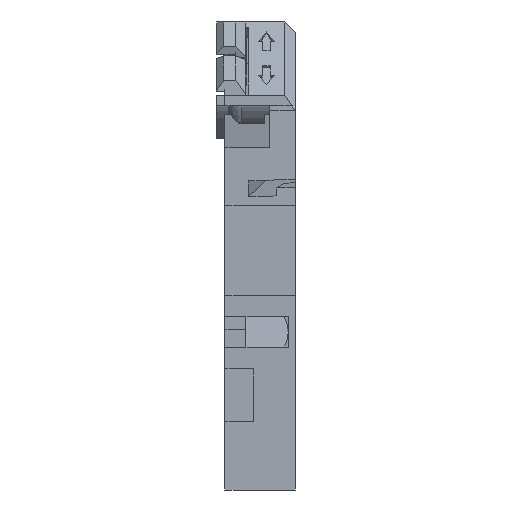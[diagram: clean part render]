
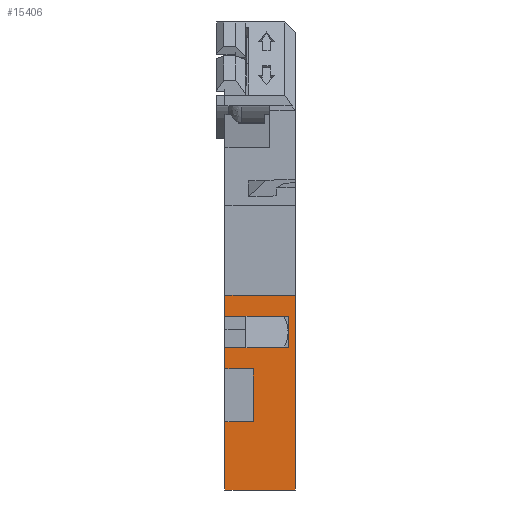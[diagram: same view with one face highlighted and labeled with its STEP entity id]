
A CAD part, left-side view. The second image highlights one B-rep face of the part: STEP entity #15406.
In plain terms, the highlighted planar face has unit normal (-1, 0, 0).
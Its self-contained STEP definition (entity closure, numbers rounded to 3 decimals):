
#14422 = VERTEX_POINT('',#14423);
#14423 = CARTESIAN_POINT('',(-50.,-1.6,-40.));
#14429 = EDGE_CURVE('',#14422,#14430,#14432,.T.);
#14430 = VERTEX_POINT('',#14431);
#14431 = CARTESIAN_POINT('',(-50.,-1.6,-27.));
#14432 = LINE('',#14433,#14434);
#14433 = CARTESIAN_POINT('',(-50.,-1.6,-40.));
#14434 = VECTOR('',#14435,1.);
#14435 = DIRECTION('',(0.,0.,1.));
#14454 = VERTEX_POINT('',#14455);
#14455 = CARTESIAN_POINT('',(-50.,-1.6,-17.));
#14461 = EDGE_CURVE('',#14462,#14454,#14464,.T.);
#14462 = VERTEX_POINT('',#14463);
#14463 = CARTESIAN_POINT('',(-50.,-1.6,-13.));
#14464 = LINE('',#14465,#14466);
#14465 = CARTESIAN_POINT('',(-50.,-1.6,-13.));
#14466 = VECTOR('',#14467,1.);
#14467 = DIRECTION('',(0.,0.,-1.));
#15386 = EDGE_CURVE('',#14422,#15387,#15389,.T.);
#15387 = VERTEX_POINT('',#15388);
#15388 = CARTESIAN_POINT('',(-50.,-15.,-40.));
#15389 = LINE('',#15390,#15391);
#15390 = CARTESIAN_POINT('',(-50.,0.,-40.));
#15391 = VECTOR('',#15392,1.);
#15392 = DIRECTION('',(0.,-1.,0.));
#15406 = ADVANCED_FACE('',(#15407),#15480,.T.);
#15407 = FACE_BOUND('',#15408,.T.);
#15408 = EDGE_LOOP('',(#15409,#15419,#15425,#15426,#15427,#15435,#15443,
    #15451,#15459,#15467,#15473,#15474));
#15409 = ORIENTED_EDGE('',*,*,#15410,.F.);
#15410 = EDGE_CURVE('',#15411,#15413,#15415,.T.);
#15411 = VERTEX_POINT('',#15412);
#15412 = CARTESIAN_POINT('',(-50.,-7.,-27.));
#15413 = VERTEX_POINT('',#15414);
#15414 = CARTESIAN_POINT('',(-50.,-7.,-17.));
#15415 = LINE('',#15416,#15417);
#15416 = CARTESIAN_POINT('',(-50.,-7.,-27.));
#15417 = VECTOR('',#15418,1.);
#15418 = DIRECTION('',(0.,0.,1.));
#15419 = ORIENTED_EDGE('',*,*,#15420,.F.);
#15420 = EDGE_CURVE('',#14430,#15411,#15421,.T.);
#15421 = LINE('',#15422,#15423);
#15422 = CARTESIAN_POINT('',(-50.,0.,-27.));
#15423 = VECTOR('',#15424,1.);
#15424 = DIRECTION('',(0.,-1.,0.));
#15425 = ORIENTED_EDGE('',*,*,#14429,.F.);
#15426 = ORIENTED_EDGE('',*,*,#15386,.T.);
#15427 = ORIENTED_EDGE('',*,*,#15428,.F.);
#15428 = EDGE_CURVE('',#15429,#15387,#15431,.T.);
#15429 = VERTEX_POINT('',#15430);
#15430 = CARTESIAN_POINT('',(-50.,-15.,-3.));
#15431 = LINE('',#15432,#15433);
#15432 = CARTESIAN_POINT('',(-50.,-15.,33.));
#15433 = VECTOR('',#15434,1.);
#15434 = DIRECTION('',(0.,0.,-1.));
#15435 = ORIENTED_EDGE('',*,*,#15436,.F.);
#15436 = EDGE_CURVE('',#15437,#15429,#15439,.T.);
#15437 = VERTEX_POINT('',#15438);
#15438 = CARTESIAN_POINT('',(-50.,-1.6,-3.));
#15439 = LINE('',#15440,#15441);
#15440 = CARTESIAN_POINT('',(-50.,0.,-3.));
#15441 = VECTOR('',#15442,1.);
#15442 = DIRECTION('',(0.,-1.,0.));
#15443 = ORIENTED_EDGE('',*,*,#15444,.F.);
#15444 = EDGE_CURVE('',#15445,#15437,#15447,.T.);
#15445 = VERTEX_POINT('',#15446);
#15446 = CARTESIAN_POINT('',(-50.,-1.6,-7.));
#15447 = LINE('',#15448,#15449);
#15448 = CARTESIAN_POINT('',(-50.,-1.6,-40.));
#15449 = VECTOR('',#15450,1.);
#15450 = DIRECTION('',(0.,0.,1.));
#15451 = ORIENTED_EDGE('',*,*,#15452,.F.);
#15452 = EDGE_CURVE('',#15453,#15445,#15455,.T.);
#15453 = VERTEX_POINT('',#15454);
#15454 = CARTESIAN_POINT('',(-50.,-13.6,-7.));
#15455 = LINE('',#15456,#15457);
#15456 = CARTESIAN_POINT('',(-50.,-15.,-7.));
#15457 = VECTOR('',#15458,1.);
#15458 = DIRECTION('',(0.,1.,0.));
#15459 = ORIENTED_EDGE('',*,*,#15460,.T.);
#15460 = EDGE_CURVE('',#15453,#15461,#15463,.T.);
#15461 = VERTEX_POINT('',#15462);
#15462 = CARTESIAN_POINT('',(-50.,-13.6,-13.));
#15463 = LINE('',#15464,#15465);
#15464 = CARTESIAN_POINT('',(-50.,-13.6,-5.));
#15465 = VECTOR('',#15466,1.);
#15466 = DIRECTION('',(0.,0.,-1.));
#15467 = ORIENTED_EDGE('',*,*,#15468,.T.);
#15468 = EDGE_CURVE('',#15461,#14462,#15469,.T.);
#15469 = LINE('',#15470,#15471);
#15470 = CARTESIAN_POINT('',(-50.,-15.,-13.));
#15471 = VECTOR('',#15472,1.);
#15472 = DIRECTION('',(0.,1.,0.));
#15473 = ORIENTED_EDGE('',*,*,#14461,.T.);
#15474 = ORIENTED_EDGE('',*,*,#15475,.T.);
#15475 = EDGE_CURVE('',#14454,#15413,#15476,.T.);
#15476 = LINE('',#15477,#15478);
#15477 = CARTESIAN_POINT('',(-50.,0.,-17.));
#15478 = VECTOR('',#15479,1.);
#15479 = DIRECTION('',(0.,-1.,0.));
#15480 = PLANE('',#15481);
#15481 = AXIS2_PLACEMENT_3D('',#15482,#15483,#15484);
#15482 = CARTESIAN_POINT('',(-50.,-8.787,-19.504));
#15483 = DIRECTION('',(-1.,0.,0.));
#15484 = DIRECTION('',(0.,1.,0.));
